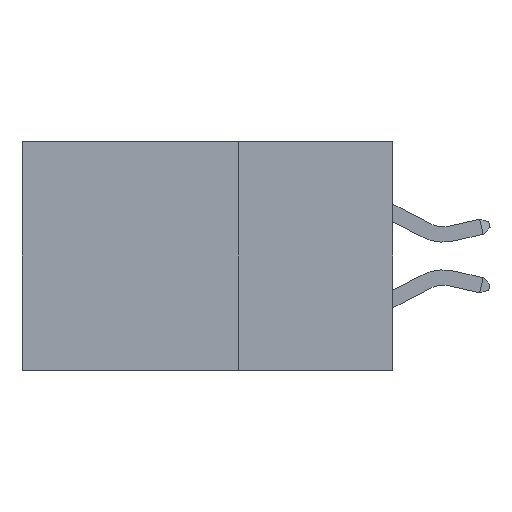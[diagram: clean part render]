
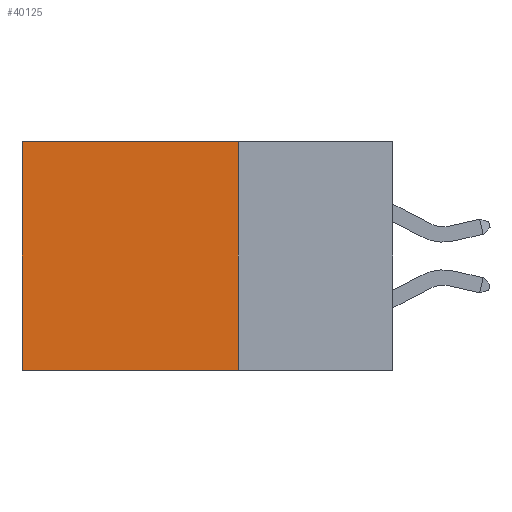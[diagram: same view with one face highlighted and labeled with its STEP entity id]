
A CAD part, left-side view. The second image highlights one B-rep face of the part: STEP entity #40125.
In plain terms, the highlighted planar face has unit normal (-1, 0, 0).
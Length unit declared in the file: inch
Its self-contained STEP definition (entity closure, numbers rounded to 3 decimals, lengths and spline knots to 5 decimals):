
#280 = CARTESIAN_POINT ( 'NONE',  ( 0.2875, 0.25, -0.37 ) ) ;
#1248 = DIRECTION ( 'NONE',  ( 0., 0., -1. ) ) ;
#3633 = DIRECTION ( 'NONE',  ( 0., 1., 0. ) ) ;
#4443 = CARTESIAN_POINT ( 'NONE',  ( 0.2875, 0.6, -0.37 ) ) ;
#6403 = DIRECTION ( 'NONE',  ( 1., 0., 0. ) ) ;
#6968 = LINE ( 'NONE', #280, #41359 ) ;
#7848 = EDGE_CURVE ( 'NONE', #24564, #12837, #6968, .T. ) ;
#8289 = ORIENTED_EDGE ( 'NONE', *, *, #17612, .T. ) ;
#8930 = DIRECTION ( 'NONE',  ( 0., 1., 0. ) ) ;
#9514 = FACE_OUTER_BOUND ( 'NONE', #13060, .T. ) ;
#10414 = CARTESIAN_POINT ( 'NONE',  ( 0.2875, 0.25, 0. ) ) ;
#10873 = CARTESIAN_POINT ( 'NONE',  ( 0.2875, 0.25, -0.37 ) ) ;
#12837 = VERTEX_POINT ( 'NONE', #4443 ) ;
#13060 = EDGE_LOOP ( 'NONE', ( #43478, #37991, #31611, #8289 ) ) ;
#14186 = LINE ( 'NONE', #10414, #18398 ) ;
#14713 = VECTOR ( 'NONE', #8930, 39.37008 ) ;
#16204 = PLANE ( 'NONE',  #33518 ) ;
#17612 = EDGE_CURVE ( 'NONE', #25711, #17705, #28981, .T. ) ;
#17705 = VERTEX_POINT ( 'NONE', #20278 ) ;
#18282 = EDGE_CURVE ( 'NONE', #25711, #24564, #14186, .T. ) ;
#18398 = VECTOR ( 'NONE', #24657, 39.37008 ) ;
#20278 = CARTESIAN_POINT ( 'NONE',  ( 0.2875, 0.6, 0. ) ) ;
#24564 = VERTEX_POINT ( 'NONE', #10873 ) ;
#24657 = DIRECTION ( 'NONE',  ( 0., 0., -1. ) ) ;
#25711 = VERTEX_POINT ( 'NONE', #33190 ) ;
#26007 = DIRECTION ( 'NONE',  ( 0., 0., -1. ) ) ;
#28981 = LINE ( 'NONE', #39462, #14713 ) ;
#31611 = ORIENTED_EDGE ( 'NONE', *, *, #18282, .F. ) ;
#33190 = CARTESIAN_POINT ( 'NONE',  ( 0.2875, 0.25, 0. ) ) ;
#33518 = AXIS2_PLACEMENT_3D ( 'NONE', #33575, #6403, #26007 ) ;
#33575 = CARTESIAN_POINT ( 'NONE',  ( 0.2875, 0.25, 0. ) ) ;
#35524 = CARTESIAN_POINT ( 'NONE',  ( 0.2875, 0.6, 0. ) ) ;
#36993 = EDGE_CURVE ( 'NONE', #17705, #12837, #39334, .T. ) ;
#37991 = ORIENTED_EDGE ( 'NONE', *, *, #7848, .F. ) ;
#39334 = LINE ( 'NONE', #35524, #43470 ) ;
#39462 = CARTESIAN_POINT ( 'NONE',  ( 0.2875, 0.25, 0. ) ) ;
#40125 = ADVANCED_FACE ( 'NONE', ( #9514 ), #16204, .F. ) ;
#41359 = VECTOR ( 'NONE', #3633, 39.37008 ) ;
#43470 = VECTOR ( 'NONE', #1248, 39.37008 ) ;
#43478 = ORIENTED_EDGE ( 'NONE', *, *, #36993, .T. ) ;
